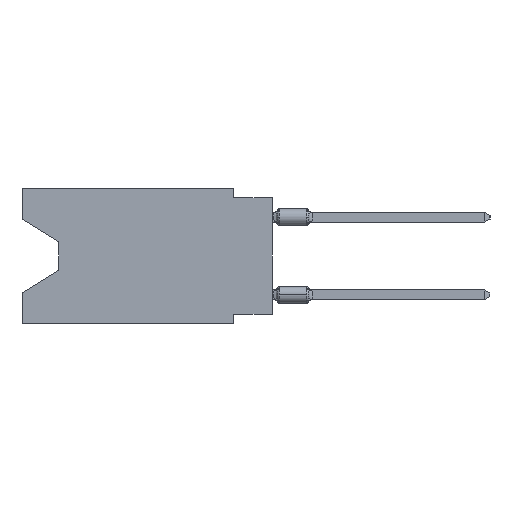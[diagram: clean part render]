
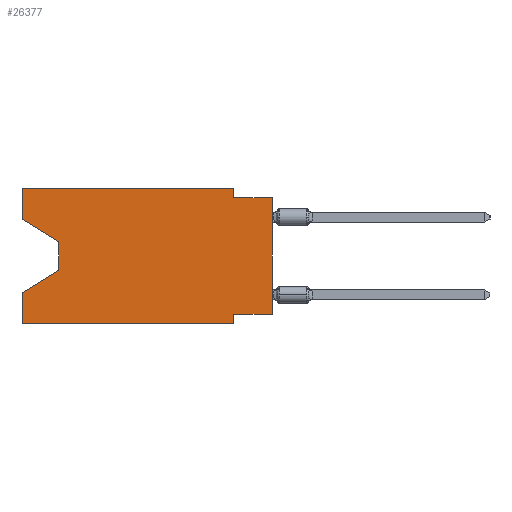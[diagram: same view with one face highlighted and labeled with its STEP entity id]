
A CAD part, left-side view. The second image highlights one B-rep face of the part: STEP entity #26377.
In plain terms, the highlighted planar face has unit normal (-1, 0, 0).
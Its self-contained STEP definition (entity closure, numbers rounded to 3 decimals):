
#310 = VERTEX_POINT ( 'NONE', #39623 ) ;
#924 = VECTOR ( 'NONE', #49843, 1000. ) ;
#1232 = DIRECTION ( 'NONE',  ( 0., -1., 0. ) ) ;
#2186 = LINE ( 'NONE', #16004, #40486 ) ;
#2372 = EDGE_CURVE ( 'NONE', #39270, #53921, #26294, .T. ) ;
#4227 = VECTOR ( 'NONE', #13644, 1000. ) ;
#5431 = VECTOR ( 'NONE', #1232, 1000. ) ;
#5433 = DIRECTION ( 'NONE',  ( 0., 0., -1. ) ) ;
#7386 = ORIENTED_EDGE ( 'NONE', *, *, #38828, .T. ) ;
#8241 = CARTESIAN_POINT ( 'NONE',  ( 0., 16.383, -8.89 ) ) ;
#8974 = LINE ( 'NONE', #23395, #32614 ) ;
#9170 = EDGE_CURVE ( 'NONE', #24187, #48113, #51414, .T. ) ;
#9277 = CARTESIAN_POINT ( 'NONE',  ( 0., 16.383, 0. ) ) ;
#9798 = EDGE_CURVE ( 'NONE', #23540, #310, #28807, .T. ) ;
#10349 = CARTESIAN_POINT ( 'NONE',  ( 0., 16.383, 0. ) ) ;
#12200 = ORIENTED_EDGE ( 'NONE', *, *, #21882, .F. ) ;
#12911 = CARTESIAN_POINT ( 'NONE',  ( 0., 13.97, -3.505 ) ) ;
#13644 = DIRECTION ( 'NONE',  ( 0., 0.855, -0.519 ) ) ;
#14183 = AXIS2_PLACEMENT_3D ( 'NONE', #34528, #37352, #52873 ) ;
#14844 = VERTEX_POINT ( 'NONE', #31358 ) ;
#14881 = VECTOR ( 'NONE', #34722, 1000. ) ;
#15274 = CARTESIAN_POINT ( 'NONE',  ( 0., 0., 0. ) ) ;
#16004 = CARTESIAN_POINT ( 'NONE',  ( 0., 2.54, -8.89 ) ) ;
#17534 = DIRECTION ( 'NONE',  ( 0., -0.855, -0.519 ) ) ;
#17636 = CARTESIAN_POINT ( 'NONE',  ( 0., 16.383, -8.89 ) ) ;
#18070 = EDGE_CURVE ( 'NONE', #58186, #47266, #51061, .T. ) ;
#18308 = LINE ( 'NONE', #12911, #55081 ) ;
#18478 = DIRECTION ( 'NONE',  ( 0., -1., 0. ) ) ;
#18700 = CARTESIAN_POINT ( 'NONE',  ( 0., 2.54, -8.89 ) ) ;
#19274 = VECTOR ( 'NONE', #18478, 1000. ) ;
#19558 = CARTESIAN_POINT ( 'NONE',  ( 0., 2.54, 0. ) ) ;
#19609 = DIRECTION ( 'NONE',  ( 0., 1., 0. ) ) ;
#20522 = DIRECTION ( 'NONE',  ( 0., 0., -1. ) ) ;
#21486 = ORIENTED_EDGE ( 'NONE', *, *, #32255, .T. ) ;
#21882 = EDGE_CURVE ( 'NONE', #39270, #14844, #8974, .T. ) ;
#22774 = DIRECTION ( 'NONE',  ( 0., 0., 1. ) ) ;
#23395 = CARTESIAN_POINT ( 'NONE',  ( 0., 16.383, 0. ) ) ;
#23540 = VERTEX_POINT ( 'NONE', #48362 ) ;
#23828 = CARTESIAN_POINT ( 'NONE',  ( 0., 13.97, -5.385 ) ) ;
#24187 = VERTEX_POINT ( 'NONE', #31415 ) ;
#24281 = ORIENTED_EDGE ( 'NONE', *, *, #52871, .T. ) ;
#24429 = EDGE_LOOP ( 'NONE', ( #24281, #7386, #21486, #12200, #24551, #44132, #45105, #25645, #57317, #36271, #44098, #33767 ) ) ;
#24551 = ORIENTED_EDGE ( 'NONE', *, *, #2372, .T. ) ;
#25645 = ORIENTED_EDGE ( 'NONE', *, *, #9798, .T. ) ;
#26294 = LINE ( 'NONE', #8241, #14881 ) ;
#26377 = ADVANCED_FACE ( 'NONE', ( #57393 ), #29749, .F. ) ;
#28807 = LINE ( 'NONE', #15274, #38537 ) ;
#29749 = PLANE ( 'NONE',  #14183 ) ;
#29847 = CARTESIAN_POINT ( 'NONE',  ( 0., 13.97, -3.505 ) ) ;
#30219 = EDGE_CURVE ( 'NONE', #48113, #310, #42430, .T. ) ;
#31358 = CARTESIAN_POINT ( 'NONE',  ( 0., 16.383, -6.852 ) ) ;
#31415 = CARTESIAN_POINT ( 'NONE',  ( 0., 2.54, 0. ) ) ;
#32255 = EDGE_CURVE ( 'NONE', #34276, #14844, #46666, .T. ) ;
#32440 = EDGE_CURVE ( 'NONE', #23540, #53214, #56572, .T. ) ;
#32614 = VECTOR ( 'NONE', #22774, 1000. ) ;
#33767 = ORIENTED_EDGE ( 'NONE', *, *, #18070, .F. ) ;
#34015 = CARTESIAN_POINT ( 'NONE',  ( 0., 0., -8.255 ) ) ;
#34276 = VERTEX_POINT ( 'NONE', #59184 ) ;
#34528 = CARTESIAN_POINT ( 'NONE',  ( 0., 16.383, 0. ) ) ;
#34722 = DIRECTION ( 'NONE',  ( 0., -1., 0. ) ) ;
#36131 = CARTESIAN_POINT ( 'NONE',  ( 0., 16.383, -2.038 ) ) ;
#36271 = ORIENTED_EDGE ( 'NONE', *, *, #9170, .F. ) ;
#37216 = CARTESIAN_POINT ( 'NONE',  ( 0., 16.383, 0. ) ) ;
#37352 = DIRECTION ( 'NONE',  ( 1., 0., 0. ) ) ;
#38537 = VECTOR ( 'NONE', #38709, 1000. ) ;
#38709 = DIRECTION ( 'NONE',  ( 0., 0., 1. ) ) ;
#38828 = EDGE_CURVE ( 'NONE', #42125, #34276, #18308, .T. ) ;
#39270 = VERTEX_POINT ( 'NONE', #17636 ) ;
#39623 = CARTESIAN_POINT ( 'NONE',  ( 0., 0., -0.635 ) ) ;
#40262 = VECTOR ( 'NONE', #5433, 1000. ) ;
#40486 = VECTOR ( 'NONE', #20522, 1000. ) ;
#40940 = EDGE_CURVE ( 'NONE', #47266, #24187, #46711, .T. ) ;
#41551 = CARTESIAN_POINT ( 'NONE',  ( 0., 0., -0.635 ) ) ;
#42125 = VERTEX_POINT ( 'NONE', #29847 ) ;
#42430 = LINE ( 'NONE', #41551, #5431 ) ;
#43638 = CARTESIAN_POINT ( 'NONE',  ( 0., 2.54, -8.255 ) ) ;
#44098 = ORIENTED_EDGE ( 'NONE', *, *, #40940, .F. ) ;
#44132 = ORIENTED_EDGE ( 'NONE', *, *, #58359, .F. ) ;
#45105 = ORIENTED_EDGE ( 'NONE', *, *, #32440, .F. ) ;
#45534 = CARTESIAN_POINT ( 'NONE',  ( 0., 16.383, -2.038 ) ) ;
#46666 = LINE ( 'NONE', #23828, #4227 ) ;
#46711 = LINE ( 'NONE', #10349, #19274 ) ;
#47266 = VERTEX_POINT ( 'NONE', #37216 ) ;
#47409 = VECTOR ( 'NONE', #19609, 1000. ) ;
#48113 = VERTEX_POINT ( 'NONE', #55342 ) ;
#48362 = CARTESIAN_POINT ( 'NONE',  ( 0., 0., -8.255 ) ) ;
#49843 = DIRECTION ( 'NONE',  ( 0., 0., 1. ) ) ;
#51061 = LINE ( 'NONE', #9277, #924 ) ;
#51414 = LINE ( 'NONE', #19558, #40262 ) ;
#52871 = EDGE_CURVE ( 'NONE', #58186, #42125, #58724, .T. ) ;
#52873 = DIRECTION ( 'NONE',  ( 0., 0., -1. ) ) ;
#53214 = VERTEX_POINT ( 'NONE', #43638 ) ;
#53921 = VERTEX_POINT ( 'NONE', #18700 ) ;
#54657 = VECTOR ( 'NONE', #17534, 1000. ) ;
#54678 = DIRECTION ( 'NONE',  ( 0., 0., -1. ) ) ;
#55081 = VECTOR ( 'NONE', #54678, 1000. ) ;
#55342 = CARTESIAN_POINT ( 'NONE',  ( 0., 2.54, -0.635 ) ) ;
#56572 = LINE ( 'NONE', #34015, #47409 ) ;
#57317 = ORIENTED_EDGE ( 'NONE', *, *, #30219, .F. ) ;
#57393 = FACE_OUTER_BOUND ( 'NONE', #24429, .T. ) ;
#58186 = VERTEX_POINT ( 'NONE', #45534 ) ;
#58359 = EDGE_CURVE ( 'NONE', #53214, #53921, #2186, .T. ) ;
#58724 = LINE ( 'NONE', #36131, #54657 ) ;
#59184 = CARTESIAN_POINT ( 'NONE',  ( 0., 13.97, -5.385 ) ) ;
